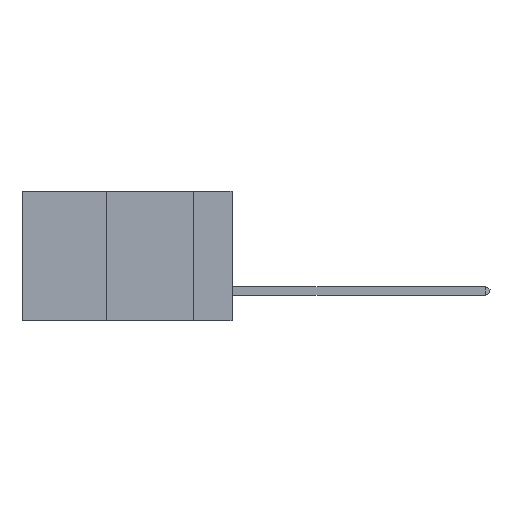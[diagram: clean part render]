
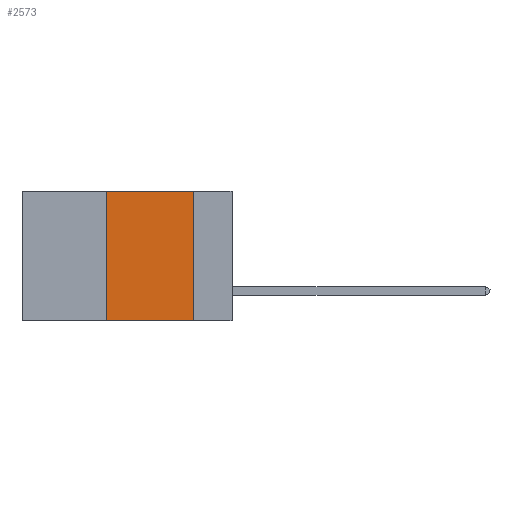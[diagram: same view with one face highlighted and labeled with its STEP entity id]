
A CAD part, left-side view. The second image highlights one B-rep face of the part: STEP entity #2573.
In plain terms, the highlighted planar face has unit normal (-1, 0, 0).
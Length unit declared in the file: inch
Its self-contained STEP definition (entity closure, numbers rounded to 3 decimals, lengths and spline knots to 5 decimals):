
#275 = EDGE_LOOP ( 'NONE', ( #10238, #1963, #10923, #12517 ) ) ;
#314 = CARTESIAN_POINT ( 'NONE',  ( 0., 0.36, -0.37 ) ) ;
#623 = CARTESIAN_POINT ( 'NONE',  ( 0., 0.36, 0. ) ) ;
#660 = LINE ( 'NONE', #6606, #10033 ) ;
#1052 = LINE ( 'NONE', #7003, #7037 ) ;
#1690 = DIRECTION ( 'NONE',  ( 0., -1., 0. ) ) ;
#1740 = EDGE_CURVE ( 'NONE', #10404, #8210, #10981, .T. ) ;
#1963 = ORIENTED_EDGE ( 'NONE', *, *, #1740, .F. ) ;
#2038 = AXIS2_PLACEMENT_3D ( 'NONE', #13631, #6740, #11015 ) ;
#2049 = CARTESIAN_POINT ( 'NONE',  ( 0., 0.11, 0. ) ) ;
#2489 = VECTOR ( 'NONE', #7072, 39.37008 ) ;
#2573 = ADVANCED_FACE ( 'NONE', ( #2961 ), #12333, .F. ) ;
#2961 = FACE_OUTER_BOUND ( 'NONE', #275, .T. ) ;
#4820 = VECTOR ( 'NONE', #11519, 39.37008 ) ;
#6121 = EDGE_CURVE ( 'NONE', #9481, #7047, #1052, .T. ) ;
#6606 = CARTESIAN_POINT ( 'NONE',  ( 0., 0.11, 0. ) ) ;
#6740 = DIRECTION ( 'NONE',  ( 1., 0., 0. ) ) ;
#7003 = CARTESIAN_POINT ( 'NONE',  ( 0., 0.6, -0.37 ) ) ;
#7037 = VECTOR ( 'NONE', #1690, 39.37008 ) ;
#7047 = VERTEX_POINT ( 'NONE', #10382 ) ;
#7072 = DIRECTION ( 'NONE',  ( 0., 0., 1. ) ) ;
#7413 = CARTESIAN_POINT ( 'NONE',  ( 0., 0.6, 0. ) ) ;
#7776 = DIRECTION ( 'NONE',  ( 0., 0., -1. ) ) ;
#8157 = EDGE_CURVE ( 'NONE', #9481, #10404, #9868, .T. ) ;
#8210 = VERTEX_POINT ( 'NONE', #2049 ) ;
#8385 = EDGE_CURVE ( 'NONE', #8210, #7047, #660, .T. ) ;
#9481 = VERTEX_POINT ( 'NONE', #314 ) ;
#9868 = LINE ( 'NONE', #10364, #2489 ) ;
#10033 = VECTOR ( 'NONE', #7776, 39.37008 ) ;
#10238 = ORIENTED_EDGE ( 'NONE', *, *, #8385, .F. ) ;
#10364 = CARTESIAN_POINT ( 'NONE',  ( 0., 0.36, 0. ) ) ;
#10382 = CARTESIAN_POINT ( 'NONE',  ( 0., 0.11, -0.37 ) ) ;
#10404 = VERTEX_POINT ( 'NONE', #623 ) ;
#10923 = ORIENTED_EDGE ( 'NONE', *, *, #8157, .F. ) ;
#10981 = LINE ( 'NONE', #7413, #4820 ) ;
#11015 = DIRECTION ( 'NONE',  ( 0., 0., -1. ) ) ;
#11519 = DIRECTION ( 'NONE',  ( 0., -1., 0. ) ) ;
#12333 = PLANE ( 'NONE',  #2038 ) ;
#12517 = ORIENTED_EDGE ( 'NONE', *, *, #6121, .T. ) ;
#13631 = CARTESIAN_POINT ( 'NONE',  ( 0., 0.6, 0. ) ) ;
